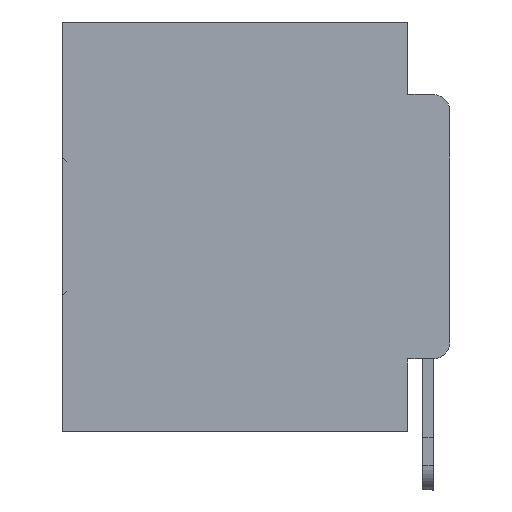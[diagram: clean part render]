
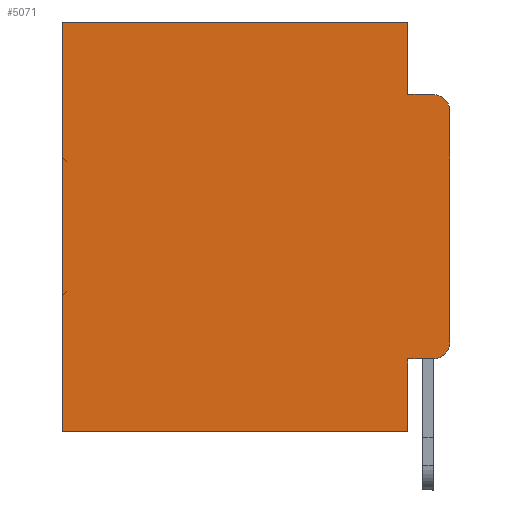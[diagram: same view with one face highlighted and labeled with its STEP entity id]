
A CAD part, left-side view. The second image highlights one B-rep face of the part: STEP entity #5071.
In plain terms, the highlighted planar face has unit normal (-1, 0, 0).
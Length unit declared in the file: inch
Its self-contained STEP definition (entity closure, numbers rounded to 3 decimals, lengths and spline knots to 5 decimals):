
#24 = LINE ( 'NONE', #10461, #13785 ) ;
#53 = VERTEX_POINT ( 'NONE', #14115 ) ;
#65 = EDGE_CURVE ( 'NONE', #1420, #3504, #8395, .T. ) ;
#243 = VERTEX_POINT ( 'NONE', #7608 ) ;
#591 = LINE ( 'NONE', #32361, #25122 ) ;
#808 = DIRECTION ( 'NONE',  ( 0., 0., -1. ) ) ;
#1420 = VERTEX_POINT ( 'NONE', #6473 ) ;
#1431 = DIRECTION ( 'NONE',  ( 0., -1., 0. ) ) ;
#1730 = CARTESIAN_POINT ( 'NONE',  ( 0.298, 0.473, -0.5 ) ) ;
#2031 = CARTESIAN_POINT ( 'NONE',  ( 0.298, 0., -0.5 ) ) ;
#2390 = AXIS2_PLACEMENT_3D ( 'NONE', #11900, #12246, #6937 ) ;
#2851 = EDGE_CURVE ( 'NONE', #1420, #14372, #26585, .T. ) ;
#3228 = CARTESIAN_POINT ( 'NONE',  ( 0.298, 0.051, 0. ) ) ;
#3504 = VERTEX_POINT ( 'NONE', #4305 ) ;
#3641 = DIRECTION ( 'NONE',  ( 0., 0., -1. ) ) ;
#4305 = CARTESIAN_POINT ( 'NONE',  ( 0.298, 0.02, -0.0885 ) ) ;
#4316 = VERTEX_POINT ( 'NONE', #1730 ) ;
#5032 = PLANE ( 'NONE',  #17002 ) ;
#5071 = ADVANCED_FACE ( 'NONE', ( #30498 ), #5032, .F. ) ;
#5421 = VECTOR ( 'NONE', #25210, 39.37008 ) ;
#5924 = CARTESIAN_POINT ( 'NONE',  ( 0.298, 0., 0. ) ) ;
#6146 = VECTOR ( 'NONE', #28458, 39.37008 ) ;
#6473 = CARTESIAN_POINT ( 'NONE',  ( 0.298, 0., -0.1085 ) ) ;
#6919 = DIRECTION ( 'NONE',  ( 0., 1., 0. ) ) ;
#6937 = DIRECTION ( 'NONE',  ( 0., 0., -1. ) ) ;
#7307 = EDGE_CURVE ( 'NONE', #21374, #14372, #25619, .T. ) ;
#7608 = CARTESIAN_POINT ( 'NONE',  ( 0.298, 0.051, -0.5 ) ) ;
#8200 = EDGE_CURVE ( 'NONE', #53, #3504, #25536, .T. ) ;
#8395 = CIRCLE ( 'NONE', #2390, 0.02 ) ;
#9859 = CARTESIAN_POINT ( 'NONE',  ( 0.298, 0.051, -0.0885 ) ) ;
#10461 = CARTESIAN_POINT ( 'NONE',  ( 0.298, 0., 0. ) ) ;
#11286 = ORIENTED_EDGE ( 'NONE', *, *, #29140, .F. ) ;
#11451 = CARTESIAN_POINT ( 'NONE',  ( 0.298, 0., -0.3915 ) ) ;
#11900 = CARTESIAN_POINT ( 'NONE',  ( 0.298, 0.02, -0.1085 ) ) ;
#12148 = EDGE_CURVE ( 'NONE', #21359, #21374, #591, .T. ) ;
#12246 = DIRECTION ( 'NONE',  ( -1., 0., 0. ) ) ;
#13191 = ORIENTED_EDGE ( 'NONE', *, *, #31309, .T. ) ;
#13652 = VECTOR ( 'NONE', #30887, 39.37008 ) ;
#13785 = VECTOR ( 'NONE', #6919, 39.37008 ) ;
#14115 = CARTESIAN_POINT ( 'NONE',  ( 0.298, 0.051, -0.0885 ) ) ;
#14372 = VERTEX_POINT ( 'NONE', #11451 ) ;
#14474 = DIRECTION ( 'NONE',  ( 1., 0., 0. ) ) ;
#14532 = VERTEX_POINT ( 'NONE', #31234 ) ;
#15267 = AXIS2_PLACEMENT_3D ( 'NONE', #17903, #33623, #25263 ) ;
#15495 = ORIENTED_EDGE ( 'NONE', *, *, #65, .T. ) ;
#16043 = DIRECTION ( 'NONE',  ( 0., 0., -1. ) ) ;
#16190 = ORIENTED_EDGE ( 'NONE', *, *, #19091, .F. ) ;
#16773 = ORIENTED_EDGE ( 'NONE', *, *, #31050, .T. ) ;
#16909 = EDGE_CURVE ( 'NONE', #21359, #243, #26859, .T. ) ;
#17002 = AXIS2_PLACEMENT_3D ( 'NONE', #20076, #14474, #17187 ) ;
#17187 = DIRECTION ( 'NONE',  ( 0., 0., -1. ) ) ;
#17835 = ORIENTED_EDGE ( 'NONE', *, *, #7307, .T. ) ;
#17903 = CARTESIAN_POINT ( 'NONE',  ( 0.298, 0.02, -0.3915 ) ) ;
#18534 = CARTESIAN_POINT ( 'NONE',  ( 0.298, 0.473, 0. ) ) ;
#18676 = CARTESIAN_POINT ( 'NONE',  ( 0.298, 0.051, 0. ) ) ;
#18765 = CARTESIAN_POINT ( 'NONE',  ( 0.298, 0.051, 0. ) ) ;
#19091 = EDGE_CURVE ( 'NONE', #21189, #53, #29186, .T. ) ;
#19979 = ORIENTED_EDGE ( 'NONE', *, *, #16909, .F. ) ;
#20076 = CARTESIAN_POINT ( 'NONE',  ( 0.298, 0., 0. ) ) ;
#20150 = ORIENTED_EDGE ( 'NONE', *, *, #2851, .F. ) ;
#20513 = VECTOR ( 'NONE', #808, 39.37008 ) ;
#20780 = VECTOR ( 'NONE', #3641, 39.37008 ) ;
#21099 = LINE ( 'NONE', #18534, #6146 ) ;
#21189 = VERTEX_POINT ( 'NONE', #18765 ) ;
#21359 = VERTEX_POINT ( 'NONE', #24555 ) ;
#21374 = VERTEX_POINT ( 'NONE', #29686 ) ;
#22589 = ORIENTED_EDGE ( 'NONE', *, *, #8200, .F. ) ;
#23642 = ORIENTED_EDGE ( 'NONE', *, *, #12148, .T. ) ;
#24555 = CARTESIAN_POINT ( 'NONE',  ( 0.298, 0.051, -0.4115 ) ) ;
#25122 = VECTOR ( 'NONE', #1431, 39.37008 ) ;
#25210 = DIRECTION ( 'NONE',  ( 0., -1., 0. ) ) ;
#25263 = DIRECTION ( 'NONE',  ( 0., 0., -1. ) ) ;
#25536 = LINE ( 'NONE', #9859, #5421 ) ;
#25619 = CIRCLE ( 'NONE', #15267, 0.02 ) ;
#26585 = LINE ( 'NONE', #5924, #20513 ) ;
#26859 = LINE ( 'NONE', #18676, #20780 ) ;
#27621 = VECTOR ( 'NONE', #16043, 39.37008 ) ;
#28458 = DIRECTION ( 'NONE',  ( 0., 0., -1. ) ) ;
#29140 = EDGE_CURVE ( 'NONE', #243, #4316, #33461, .T. ) ;
#29186 = LINE ( 'NONE', #3228, #27621 ) ;
#29686 = CARTESIAN_POINT ( 'NONE',  ( 0.298, 0.02, -0.4115 ) ) ;
#30498 = FACE_OUTER_BOUND ( 'NONE', #31132, .T. ) ;
#30887 = DIRECTION ( 'NONE',  ( 0., 1., 0. ) ) ;
#31050 = EDGE_CURVE ( 'NONE', #14532, #4316, #21099, .T. ) ;
#31132 = EDGE_LOOP ( 'NONE', ( #20150, #15495, #22589, #16190, #13191, #16773, #11286, #19979, #23642, #17835 ) ) ;
#31234 = CARTESIAN_POINT ( 'NONE',  ( 0.298, 0.473, 0. ) ) ;
#31309 = EDGE_CURVE ( 'NONE', #21189, #14532, #24, .T. ) ;
#32361 = CARTESIAN_POINT ( 'NONE',  ( 0.298, 0.051, -0.4115 ) ) ;
#33461 = LINE ( 'NONE', #2031, #13652 ) ;
#33623 = DIRECTION ( 'NONE',  ( -1., 0., 0. ) ) ;
